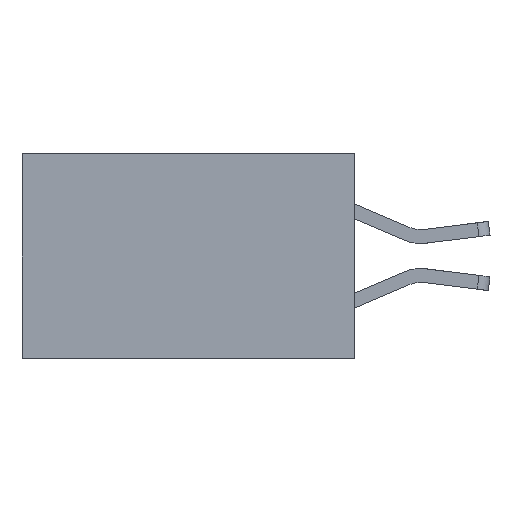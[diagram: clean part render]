
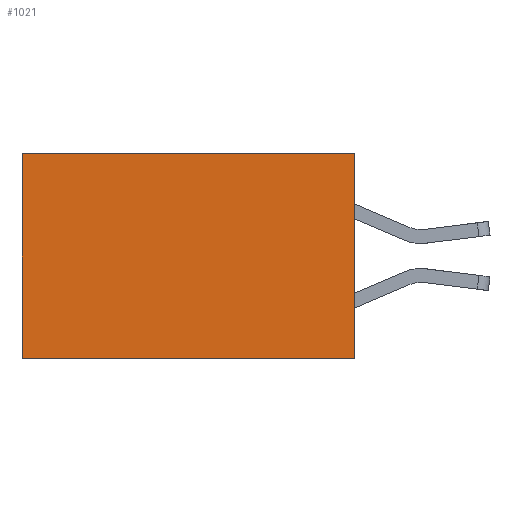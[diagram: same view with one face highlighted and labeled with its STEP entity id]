
A CAD part, left-side view. The second image highlights one B-rep face of the part: STEP entity #1021.
In plain terms, the highlighted planar face has unit normal (-1, 0, 0).
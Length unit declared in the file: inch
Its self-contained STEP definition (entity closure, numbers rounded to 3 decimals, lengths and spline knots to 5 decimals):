
#163 = DIRECTION ( 'NONE',  ( 0., 0., -1. ) ) ;
#1021 = ADVANCED_FACE ( 'NONE', ( #1918 ), #6076, .F. ) ;
#1470 = CARTESIAN_POINT ( 'NONE',  ( 0.2615, 0., -0.37 ) ) ;
#1525 = CARTESIAN_POINT ( 'NONE',  ( 0.2615, 0.6, -0.37 ) ) ;
#1918 = FACE_OUTER_BOUND ( 'NONE', #4157, .T. ) ;
#2076 = AXIS2_PLACEMENT_3D ( 'NONE', #6119, #4033, #8926 ) ;
#2277 = LINE ( 'NONE', #1525, #6570 ) ;
#2611 = CARTESIAN_POINT ( 'NONE',  ( 0.2615, 0., -0.37 ) ) ;
#3522 = EDGE_CURVE ( 'NONE', #7842, #4455, #4968, .T. ) ;
#3599 = VECTOR ( 'NONE', #6439, 39.37008 ) ;
#3643 = CARTESIAN_POINT ( 'NONE',  ( 0.2615, 0.6, 0. ) ) ;
#4025 = VERTEX_POINT ( 'NONE', #8021 ) ;
#4033 = DIRECTION ( 'NONE',  ( 1., 0., 0. ) ) ;
#4157 = EDGE_LOOP ( 'NONE', ( #8371, #4262, #6947, #8358 ) ) ;
#4262 = ORIENTED_EDGE ( 'NONE', *, *, #5668, .F. ) ;
#4347 = EDGE_CURVE ( 'NONE', #7842, #4468, #8355, .T. ) ;
#4455 = VERTEX_POINT ( 'NONE', #3643 ) ;
#4468 = VERTEX_POINT ( 'NONE', #2611 ) ;
#4968 = LINE ( 'NONE', #5702, #3599 ) ;
#5538 = VECTOR ( 'NONE', #8484, 39.37008 ) ;
#5668 = EDGE_CURVE ( 'NONE', #4468, #4025, #8747, .T. ) ;
#5702 = CARTESIAN_POINT ( 'NONE',  ( 0.2615, 0., 0. ) ) ;
#5845 = DIRECTION ( 'NONE',  ( 0., 1., 0. ) ) ;
#5846 = VECTOR ( 'NONE', #5845, 39.37008 ) ;
#6076 = PLANE ( 'NONE',  #2076 ) ;
#6119 = CARTESIAN_POINT ( 'NONE',  ( 0.2615, 0., -0.37 ) ) ;
#6145 = CARTESIAN_POINT ( 'NONE',  ( 0.2615, 0., 0. ) ) ;
#6439 = DIRECTION ( 'NONE',  ( 0., 1., 0. ) ) ;
#6570 = VECTOR ( 'NONE', #163, 39.37008 ) ;
#6622 = CARTESIAN_POINT ( 'NONE',  ( 0.2615, 0., -0.37 ) ) ;
#6947 = ORIENTED_EDGE ( 'NONE', *, *, #4347, .F. ) ;
#7180 = EDGE_CURVE ( 'NONE', #4455, #4025, #2277, .T. ) ;
#7842 = VERTEX_POINT ( 'NONE', #6145 ) ;
#8021 = CARTESIAN_POINT ( 'NONE',  ( 0.2615, 0.6, -0.37 ) ) ;
#8355 = LINE ( 'NONE', #1470, #5538 ) ;
#8358 = ORIENTED_EDGE ( 'NONE', *, *, #3522, .T. ) ;
#8371 = ORIENTED_EDGE ( 'NONE', *, *, #7180, .T. ) ;
#8484 = DIRECTION ( 'NONE',  ( 0., 0., -1. ) ) ;
#8747 = LINE ( 'NONE', #6622, #5846 ) ;
#8926 = DIRECTION ( 'NONE',  ( 0., 0., -1. ) ) ;
